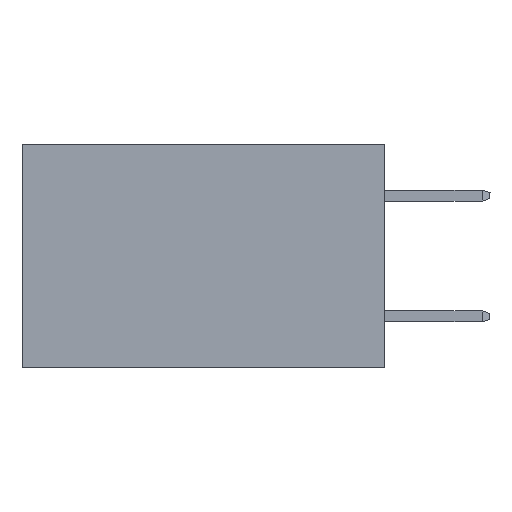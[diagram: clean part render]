
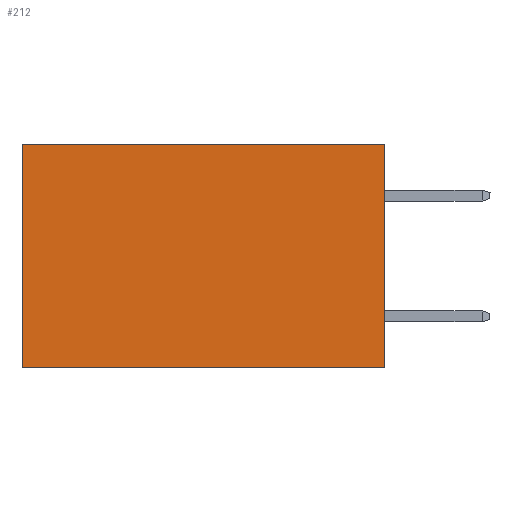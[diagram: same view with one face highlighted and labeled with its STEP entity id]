
A CAD part, left-side view. The second image highlights one B-rep face of the part: STEP entity #212.
In plain terms, the highlighted planar face has unit normal (-1, 0, 0).
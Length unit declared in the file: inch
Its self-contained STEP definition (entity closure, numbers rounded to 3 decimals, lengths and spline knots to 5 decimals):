
#212 = ADVANCED_FACE ( 'NONE', ( #5413 ), #6425, .F. ) ;
#851 = LINE ( 'NONE', #26156, #16856 ) ;
#924 = CARTESIAN_POINT ( 'NONE',  ( 0.2615, 0.6, -0.37 ) ) ;
#2277 = DIRECTION ( 'NONE',  ( 0., 0., -1. ) ) ;
#2296 = VECTOR ( 'NONE', #22603, 39.37008 ) ;
#2532 = LINE ( 'NONE', #15122, #23977 ) ;
#4134 = CARTESIAN_POINT ( 'NONE',  ( 0.2615, 0., -0.37 ) ) ;
#4414 = CARTESIAN_POINT ( 'NONE',  ( 0.2615, 0.6, -0.37 ) ) ;
#4696 = DIRECTION ( 'NONE',  ( 0., 1., 0. ) ) ;
#5103 = CARTESIAN_POINT ( 'NONE',  ( 0.2615, 0.6, 0. ) ) ;
#5413 = FACE_OUTER_BOUND ( 'NONE', #22597, .T. ) ;
#5459 = CARTESIAN_POINT ( 'NONE',  ( 0.2615, 0., -0.37 ) ) ;
#5901 = EDGE_CURVE ( 'NONE', #18598, #16042, #8548, .T. ) ;
#6425 = PLANE ( 'NONE',  #21760 ) ;
#6927 = DIRECTION ( 'NONE',  ( 1., 0., 0. ) ) ;
#8548 = LINE ( 'NONE', #20552, #2296 ) ;
#8960 = EDGE_CURVE ( 'NONE', #13305, #16042, #9767, .T. ) ;
#9767 = LINE ( 'NONE', #4414, #20131 ) ;
#9993 = EDGE_CURVE ( 'NONE', #17308, #18598, #851, .T. ) ;
#11798 = DIRECTION ( 'NONE',  ( 0., 0., -1. ) ) ;
#13305 = VERTEX_POINT ( 'NONE', #5103 ) ;
#13945 = ORIENTED_EDGE ( 'NONE', *, *, #5901, .F. ) ;
#14509 = EDGE_CURVE ( 'NONE', #17308, #13305, #2532, .T. ) ;
#15122 = CARTESIAN_POINT ( 'NONE',  ( 0.2615, 0., 0. ) ) ;
#16042 = VERTEX_POINT ( 'NONE', #924 ) ;
#16856 = VECTOR ( 'NONE', #11798, 39.37008 ) ;
#17204 = DIRECTION ( 'NONE',  ( 0., 0., -1. ) ) ;
#17308 = VERTEX_POINT ( 'NONE', #23385 ) ;
#18598 = VERTEX_POINT ( 'NONE', #5459 ) ;
#20131 = VECTOR ( 'NONE', #2277, 39.37008 ) ;
#20552 = CARTESIAN_POINT ( 'NONE',  ( 0.2615, 0., -0.37 ) ) ;
#20832 = ORIENTED_EDGE ( 'NONE', *, *, #14509, .T. ) ;
#21760 = AXIS2_PLACEMENT_3D ( 'NONE', #4134, #6927, #17204 ) ;
#22597 = EDGE_LOOP ( 'NONE', ( #25717, #13945, #26728, #20832 ) ) ;
#22603 = DIRECTION ( 'NONE',  ( 0., 1., 0. ) ) ;
#23385 = CARTESIAN_POINT ( 'NONE',  ( 0.2615, 0., 0. ) ) ;
#23977 = VECTOR ( 'NONE', #4696, 39.37008 ) ;
#25717 = ORIENTED_EDGE ( 'NONE', *, *, #8960, .T. ) ;
#26156 = CARTESIAN_POINT ( 'NONE',  ( 0.2615, 0., -0.37 ) ) ;
#26728 = ORIENTED_EDGE ( 'NONE', *, *, #9993, .F. ) ;
